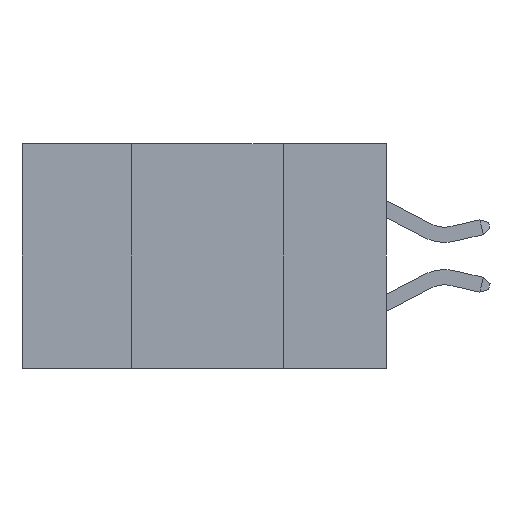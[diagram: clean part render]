
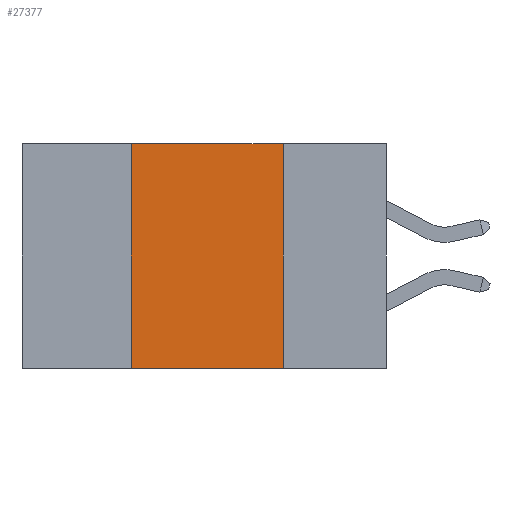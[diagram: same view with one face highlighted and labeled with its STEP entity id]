
A CAD part, left-side view. The second image highlights one B-rep face of the part: STEP entity #27377.
In plain terms, the highlighted planar face has unit normal (-1, 0, 0).
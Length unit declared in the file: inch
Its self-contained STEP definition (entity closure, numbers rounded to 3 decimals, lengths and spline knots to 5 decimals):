
#559 = VERTEX_POINT ( 'NONE', #25323 ) ;
#3626 = ORIENTED_EDGE ( 'NONE', *, *, #8892, .F. ) ;
#4429 = LINE ( 'NONE', #10410, #11783 ) ;
#5751 = CARTESIAN_POINT ( 'NONE',  ( 0., 0.17, -0.37 ) ) ;
#5776 = EDGE_CURVE ( 'NONE', #17239, #559, #9196, .T. ) ;
#6497 = ORIENTED_EDGE ( 'NONE', *, *, #21801, .F. ) ;
#7124 = EDGE_LOOP ( 'NONE', ( #6497, #3626, #18865, #11980 ) ) ;
#7646 = CARTESIAN_POINT ( 'NONE',  ( 0., 0.6, 0. ) ) ;
#8874 = FACE_OUTER_BOUND ( 'NONE', #7124, .T. ) ;
#8892 = EDGE_CURVE ( 'NONE', #559, #11275, #4429, .T. ) ;
#9196 = LINE ( 'NONE', #27413, #27650 ) ;
#9463 = LINE ( 'NONE', #20424, #25878 ) ;
#9719 = DIRECTION ( 'NONE',  ( 0., 0., -1. ) ) ;
#10410 = CARTESIAN_POINT ( 'NONE',  ( 0., 0.6, 0. ) ) ;
#10560 = CARTESIAN_POINT ( 'NONE',  ( 0., 0.6, -0.37 ) ) ;
#10806 = EDGE_CURVE ( 'NONE', #17239, #12612, #19728, .T. ) ;
#11275 = VERTEX_POINT ( 'NONE', #12946 ) ;
#11783 = VECTOR ( 'NONE', #14770, 39.37008 ) ;
#11980 = ORIENTED_EDGE ( 'NONE', *, *, #10806, .T. ) ;
#12406 = AXIS2_PLACEMENT_3D ( 'NONE', #7646, #18419, #24683 ) ;
#12612 = VERTEX_POINT ( 'NONE', #5751 ) ;
#12946 = CARTESIAN_POINT ( 'NONE',  ( 0., 0.17, 0. ) ) ;
#14256 = DIRECTION ( 'NONE',  ( 0., 0., 1. ) ) ;
#14770 = DIRECTION ( 'NONE',  ( 0., -1., 0. ) ) ;
#16758 = CARTESIAN_POINT ( 'NONE',  ( 0., 0.42, -0.37 ) ) ;
#17239 = VERTEX_POINT ( 'NONE', #16758 ) ;
#18419 = DIRECTION ( 'NONE',  ( 1., 0., 0. ) ) ;
#18865 = ORIENTED_EDGE ( 'NONE', *, *, #5776, .F. ) ;
#18902 = DIRECTION ( 'NONE',  ( 0., -1., 0. ) ) ;
#19728 = LINE ( 'NONE', #10560, #25417 ) ;
#20424 = CARTESIAN_POINT ( 'NONE',  ( 0., 0.17, 0. ) ) ;
#21801 = EDGE_CURVE ( 'NONE', #11275, #12612, #9463, .T. ) ;
#24683 = DIRECTION ( 'NONE',  ( 0., 0., -1. ) ) ;
#25323 = CARTESIAN_POINT ( 'NONE',  ( 0., 0.42, 0. ) ) ;
#25417 = VECTOR ( 'NONE', #18902, 39.37008 ) ;
#25878 = VECTOR ( 'NONE', #9719, 39.37008 ) ;
#26814 = PLANE ( 'NONE',  #12406 ) ;
#27377 = ADVANCED_FACE ( 'NONE', ( #8874 ), #26814, .F. ) ;
#27413 = CARTESIAN_POINT ( 'NONE',  ( 0., 0.42, 0. ) ) ;
#27650 = VECTOR ( 'NONE', #14256, 39.37008 ) ;
